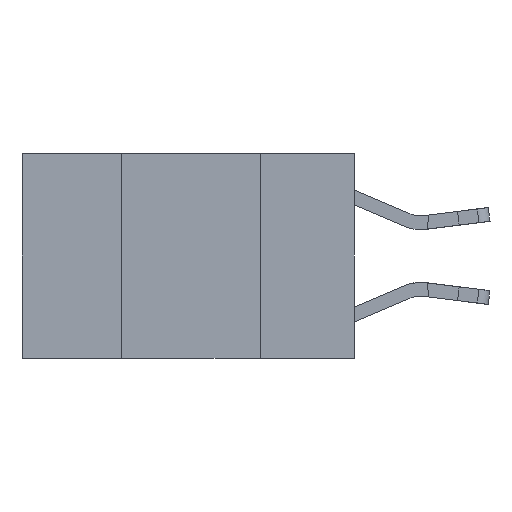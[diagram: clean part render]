
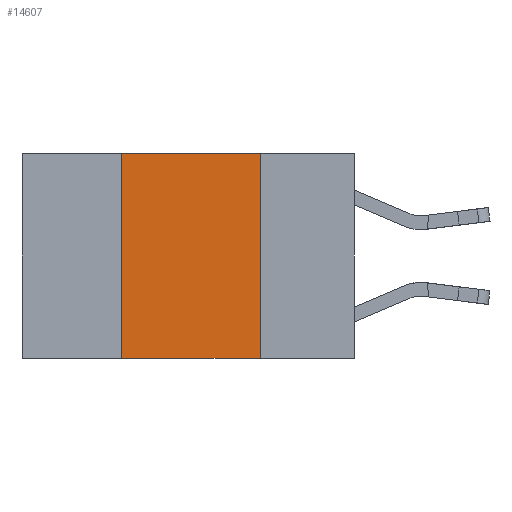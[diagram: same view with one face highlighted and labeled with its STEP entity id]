
A CAD part, left-side view. The second image highlights one B-rep face of the part: STEP entity #14607.
In plain terms, the highlighted planar face has unit normal (-1, 0, 0).
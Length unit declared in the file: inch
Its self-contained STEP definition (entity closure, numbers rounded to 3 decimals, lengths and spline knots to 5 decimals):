
#284 = VECTOR ( 'NONE', #10216, 39.37008 ) ;
#983 = VECTOR ( 'NONE', #16863, 39.37008 ) ;
#1010 = ORIENTED_EDGE ( 'NONE', *, *, #7296, .F. ) ;
#1231 = AXIS2_PLACEMENT_3D ( 'NONE', #4308, #14809, #7286 ) ;
#1849 = LINE ( 'NONE', #11933, #284 ) ;
#1894 = VECTOR ( 'NONE', #7646, 39.37008 ) ;
#2630 = ORIENTED_EDGE ( 'NONE', *, *, #16702, .F. ) ;
#3933 = CARTESIAN_POINT ( 'NONE',  ( 0., 0.42, 0. ) ) ;
#4308 = CARTESIAN_POINT ( 'NONE',  ( 0., 0.6, 0. ) ) ;
#5255 = VECTOR ( 'NONE', #5275, 39.37008 ) ;
#5275 = DIRECTION ( 'NONE',  ( 0., 0., -1. ) ) ;
#5826 = VERTEX_POINT ( 'NONE', #8003 ) ;
#6574 = VERTEX_POINT ( 'NONE', #3933 ) ;
#6625 = EDGE_CURVE ( 'NONE', #11643, #5826, #12986, .T. ) ;
#6827 = ORIENTED_EDGE ( 'NONE', *, *, #12878, .F. ) ;
#7286 = DIRECTION ( 'NONE',  ( 0., 0., -1. ) ) ;
#7296 = EDGE_CURVE ( 'NONE', #11643, #6574, #7728, .T. ) ;
#7347 = CARTESIAN_POINT ( 'NONE',  ( 0., 0.17, 0. ) ) ;
#7459 = CARTESIAN_POINT ( 'NONE',  ( 0., 0.6, -0.37 ) ) ;
#7646 = DIRECTION ( 'NONE',  ( 0., -1., 0. ) ) ;
#7728 = LINE ( 'NONE', #9366, #983 ) ;
#8003 = CARTESIAN_POINT ( 'NONE',  ( 0., 0.17, -0.37 ) ) ;
#8737 = EDGE_LOOP ( 'NONE', ( #2630, #6827, #1010, #12641 ) ) ;
#8742 = PLANE ( 'NONE',  #1231 ) ;
#9366 = CARTESIAN_POINT ( 'NONE',  ( 0., 0.42, 0. ) ) ;
#10216 = DIRECTION ( 'NONE',  ( 0., -1., 0. ) ) ;
#10641 = VERTEX_POINT ( 'NONE', #7347 ) ;
#11255 = CARTESIAN_POINT ( 'NONE',  ( 0., 0.17, 0. ) ) ;
#11643 = VERTEX_POINT ( 'NONE', #16352 ) ;
#11933 = CARTESIAN_POINT ( 'NONE',  ( 0., 0.6, 0. ) ) ;
#12641 = ORIENTED_EDGE ( 'NONE', *, *, #6625, .T. ) ;
#12878 = EDGE_CURVE ( 'NONE', #6574, #10641, #1849, .T. ) ;
#12986 = LINE ( 'NONE', #7459, #1894 ) ;
#13264 = FACE_OUTER_BOUND ( 'NONE', #8737, .T. ) ;
#14607 = ADVANCED_FACE ( 'NONE', ( #13264 ), #8742, .F. ) ;
#14809 = DIRECTION ( 'NONE',  ( 1., 0., 0. ) ) ;
#16352 = CARTESIAN_POINT ( 'NONE',  ( 0., 0.42, -0.37 ) ) ;
#16702 = EDGE_CURVE ( 'NONE', #10641, #5826, #16836, .T. ) ;
#16836 = LINE ( 'NONE', #11255, #5255 ) ;
#16863 = DIRECTION ( 'NONE',  ( 0., 0., 1. ) ) ;
